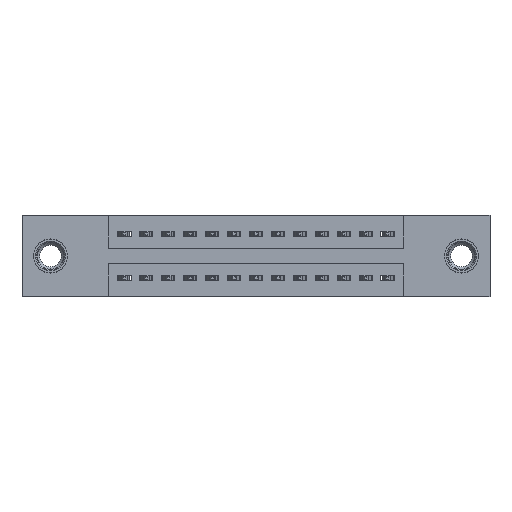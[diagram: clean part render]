
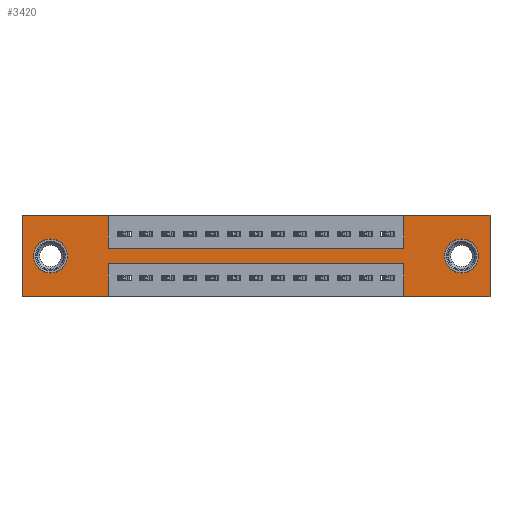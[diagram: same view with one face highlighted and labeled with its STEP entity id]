
A CAD part, front view. The second image highlights one B-rep face of the part: STEP entity #3420.
In plain terms, the highlighted planar face has unit normal (0, -1, 0).
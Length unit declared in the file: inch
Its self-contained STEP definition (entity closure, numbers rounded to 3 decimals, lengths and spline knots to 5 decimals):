
#12 = LINE ( 'NONE', #1189, #12251 ) ;
#26 = VECTOR ( 'NONE', #10800, 39.37008 ) ;
#217 = CARTESIAN_POINT ( 'NONE',  ( 0., 0., 0. ) ) ;
#230 = EDGE_CURVE ( 'NONE', #8303, #11624, #4557, .T. ) ;
#232 = ORIENTED_EDGE ( 'NONE', *, *, #5012, .F. ) ;
#518 = LINE ( 'NONE', #7254, #12726 ) ;
#530 = DIRECTION ( 'NONE',  ( -1., 0., 0. ) ) ;
#942 = CARTESIAN_POINT ( 'NONE',  ( 0.3925, 0., -0.22 ) ) ;
#1106 = VERTEX_POINT ( 'NONE', #10274 ) ;
#1141 = DIRECTION ( 'NONE',  ( 0., 0., -1. ) ) ;
#1189 = CARTESIAN_POINT ( 'NONE',  ( 1.7425, 0., 0. ) ) ;
#1346 = VERTEX_POINT ( 'NONE', #8448 ) ;
#1423 = VERTEX_POINT ( 'NONE', #8037 ) ;
#1599 = EDGE_CURVE ( 'NONE', #9933, #1677, #8602, .T. ) ;
#1677 = VERTEX_POINT ( 'NONE', #5876 ) ;
#1917 = CARTESIAN_POINT ( 'NONE',  ( 0.13, 0., -0.185 ) ) ;
#1989 = VERTEX_POINT ( 'NONE', #2842 ) ;
#2098 = ORIENTED_EDGE ( 'NONE', *, *, #14402, .F. ) ;
#2321 = EDGE_CURVE ( 'NONE', #1423, #8303, #8020, .T. ) ;
#2339 = EDGE_CURVE ( 'NONE', #1677, #9933, #11106, .T. ) ;
#2755 = DIRECTION ( 'NONE',  ( 0., 1., 0. ) ) ;
#2811 = ORIENTED_EDGE ( 'NONE', *, *, #11358, .F. ) ;
#2842 = CARTESIAN_POINT ( 'NONE',  ( 2.135, 0., -0.37 ) ) ;
#2963 = DIRECTION ( 'NONE',  ( 1., 0., 0. ) ) ;
#3110 = DIRECTION ( 'NONE',  ( 0., 0., 1. ) ) ;
#3420 = ADVANCED_FACE ( 'NONE', ( #13262, #4289, #10163 ), #3512, .T. ) ;
#3491 = AXIS2_PLACEMENT_3D ( 'NONE', #1917, #10160, #3110 ) ;
#3512 = PLANE ( 'NONE',  #15253 ) ;
#3604 = DIRECTION ( 'NONE',  ( 0., 0., 1. ) ) ;
#3617 = VERTEX_POINT ( 'NONE', #10950 ) ;
#3681 = CARTESIAN_POINT ( 'NONE',  ( 1.7425, 0., -0.22 ) ) ;
#3774 = EDGE_LOOP ( 'NONE', ( #9457, #4129 ) ) ;
#3805 = ORIENTED_EDGE ( 'NONE', *, *, #9025, .F. ) ;
#3922 = DIRECTION ( 'NONE',  ( 0., 0., -1. ) ) ;
#4040 = CARTESIAN_POINT ( 'NONE',  ( 1.7425, 0., -0.15 ) ) ;
#4041 = VECTOR ( 'NONE', #14000, 39.37008 ) ;
#4082 = CARTESIAN_POINT ( 'NONE',  ( 0., 0., 0. ) ) ;
#4129 = ORIENTED_EDGE ( 'NONE', *, *, #2339, .T. ) ;
#4289 = FACE_BOUND ( 'NONE', #5256, .T. ) ;
#4371 = AXIS2_PLACEMENT_3D ( 'NONE', #9816, #2755, #10982 ) ;
#4382 = VECTOR ( 'NONE', #5471, 39.37008 ) ;
#4389 = CARTESIAN_POINT ( 'NONE',  ( 0., 0., -0.37 ) ) ;
#4421 = DIRECTION ( 'NONE',  ( 0., 0., -1. ) ) ;
#4557 = LINE ( 'NONE', #6853, #10424 ) ;
#4796 = ORIENTED_EDGE ( 'NONE', *, *, #2321, .F. ) ;
#4852 = VERTEX_POINT ( 'NONE', #9800 ) ;
#5012 = EDGE_CURVE ( 'NONE', #4852, #1423, #7203, .T. ) ;
#5133 = ORIENTED_EDGE ( 'NONE', *, *, #12917, .F. ) ;
#5177 = VERTEX_POINT ( 'NONE', #10352 ) ;
#5256 = EDGE_LOOP ( 'NONE', ( #9571, #11284 ) ) ;
#5416 = EDGE_LOOP ( 'NONE', ( #12887, #5133, #2811, #7409, #2098, #5467, #7457, #3805, #9372, #7187, #4796, #232 ) ) ;
#5467 = ORIENTED_EDGE ( 'NONE', *, *, #10111, .F. ) ;
#5471 = DIRECTION ( 'NONE',  ( 0., 0., 1. ) ) ;
#5876 = CARTESIAN_POINT ( 'NONE',  ( 2.005, 0., -0.263 ) ) ;
#6128 = DIRECTION ( 'NONE',  ( 0., 0., -1. ) ) ;
#6266 = CARTESIAN_POINT ( 'NONE',  ( 0.13, 0., -0.185 ) ) ;
#6285 = DIRECTION ( 'NONE',  ( 0., 0., -1. ) ) ;
#6308 = DIRECTION ( 'NONE',  ( 0., 1., 0. ) ) ;
#6317 = CARTESIAN_POINT ( 'NONE',  ( 2.005, 0., -0.185 ) ) ;
#6533 = VECTOR ( 'NONE', #11842, 39.37008 ) ;
#6653 = CARTESIAN_POINT ( 'NONE',  ( 1.7425, 0., -0.37 ) ) ;
#6675 = VERTEX_POINT ( 'NONE', #942 ) ;
#6677 = VECTOR ( 'NONE', #2963, 39.37008 ) ;
#6799 = DIRECTION ( 'NONE',  ( 1., 0., 0. ) ) ;
#6853 = CARTESIAN_POINT ( 'NONE',  ( 0., 0., 0. ) ) ;
#6871 = CIRCLE ( 'NONE', #3491, 0.078 ) ;
#6905 = LINE ( 'NONE', #9526, #6533 ) ;
#7187 = ORIENTED_EDGE ( 'NONE', *, *, #230, .F. ) ;
#7189 = LINE ( 'NONE', #4389, #4041 ) ;
#7203 = LINE ( 'NONE', #14732, #13020 ) ;
#7254 = CARTESIAN_POINT ( 'NONE',  ( 0.3925, 0., 0. ) ) ;
#7409 = ORIENTED_EDGE ( 'NONE', *, *, #10504, .F. ) ;
#7411 = VERTEX_POINT ( 'NONE', #3681 ) ;
#7448 = DIRECTION ( 'NONE',  ( 0., 0., 1. ) ) ;
#7457 = ORIENTED_EDGE ( 'NONE', *, *, #10588, .F. ) ;
#7472 = EDGE_CURVE ( 'NONE', #11624, #9283, #518, .T. ) ;
#7780 = VECTOR ( 'NONE', #3922, 39.37008 ) ;
#7931 = CARTESIAN_POINT ( 'NONE',  ( 0.3925, 0., -0.37 ) ) ;
#8020 = LINE ( 'NONE', #217, #12175 ) ;
#8037 = CARTESIAN_POINT ( 'NONE',  ( 0., 0., -0.37 ) ) ;
#8189 = EDGE_CURVE ( 'NONE', #5177, #1346, #11790, .T. ) ;
#8271 = DIRECTION ( 'NONE',  ( 0., -1., 0. ) ) ;
#8303 = VERTEX_POINT ( 'NONE', #4082 ) ;
#8448 = CARTESIAN_POINT ( 'NONE',  ( 0.13, 0., -0.107 ) ) ;
#8602 = CIRCLE ( 'NONE', #12274, 0.078 ) ;
#9025 = EDGE_CURVE ( 'NONE', #9283, #12463, #10150, .T. ) ;
#9283 = VERTEX_POINT ( 'NONE', #10471 ) ;
#9372 = ORIENTED_EDGE ( 'NONE', *, *, #7472, .F. ) ;
#9457 = ORIENTED_EDGE ( 'NONE', *, *, #1599, .T. ) ;
#9526 = CARTESIAN_POINT ( 'NONE',  ( 0.3925, 0., -0.22 ) ) ;
#9571 = ORIENTED_EDGE ( 'NONE', *, *, #13810, .T. ) ;
#9641 = CARTESIAN_POINT ( 'NONE',  ( 0., 0., 0. ) ) ;
#9800 = CARTESIAN_POINT ( 'NONE',  ( 0.3925, 0., -0.37 ) ) ;
#9816 = CARTESIAN_POINT ( 'NONE',  ( 2.005, 0., -0.185 ) ) ;
#9933 = VERTEX_POINT ( 'NONE', #10455 ) ;
#10106 = VECTOR ( 'NONE', #4421, 39.37008 ) ;
#10111 = EDGE_CURVE ( 'NONE', #1106, #11264, #12636, .T. ) ;
#10115 = AXIS2_PLACEMENT_3D ( 'NONE', #6266, #14411, #7448 ) ;
#10150 = LINE ( 'NONE', #11189, #6677 ) ;
#10160 = DIRECTION ( 'NONE',  ( 0., 1., 0. ) ) ;
#10163 = FACE_OUTER_BOUND ( 'NONE', #5416, .T. ) ;
#10274 = CARTESIAN_POINT ( 'NONE',  ( 1.7425, 0., 0. ) ) ;
#10352 = CARTESIAN_POINT ( 'NONE',  ( 0.13, 0., -0.263 ) ) ;
#10424 = VECTOR ( 'NONE', #6799, 39.37008 ) ;
#10455 = CARTESIAN_POINT ( 'NONE',  ( 2.005, 0., -0.107 ) ) ;
#10471 = CARTESIAN_POINT ( 'NONE',  ( 0.3925, 0., -0.15 ) ) ;
#10504 = EDGE_CURVE ( 'NONE', #1989, #3617, #7189, .T. ) ;
#10588 = EDGE_CURVE ( 'NONE', #12463, #1106, #12, .T. ) ;
#10678 = CARTESIAN_POINT ( 'NONE',  ( 2.135, 0., 0. ) ) ;
#10682 = CARTESIAN_POINT ( 'NONE',  ( 0.3925, 0., 0. ) ) ;
#10800 = DIRECTION ( 'NONE',  ( 1., 0., 0. ) ) ;
#10864 = LINE ( 'NONE', #10942, #7780 ) ;
#10942 = CARTESIAN_POINT ( 'NONE',  ( 2.135, 0., 0. ) ) ;
#10950 = CARTESIAN_POINT ( 'NONE',  ( 1.7425, 0., -0.37 ) ) ;
#10982 = DIRECTION ( 'NONE',  ( 0., 0., -1. ) ) ;
#11106 = CIRCLE ( 'NONE', #4371, 0.078 ) ;
#11189 = CARTESIAN_POINT ( 'NONE',  ( 0.3925, 0., -0.15 ) ) ;
#11264 = VERTEX_POINT ( 'NONE', #10678 ) ;
#11284 = ORIENTED_EDGE ( 'NONE', *, *, #8189, .T. ) ;
#11358 = EDGE_CURVE ( 'NONE', #3617, #7411, #13708, .T. ) ;
#11624 = VERTEX_POINT ( 'NONE', #10682 ) ;
#11790 = CIRCLE ( 'NONE', #10115, 0.078 ) ;
#11842 = DIRECTION ( 'NONE',  ( -1., 0., 0. ) ) ;
#12034 = DIRECTION ( 'NONE',  ( 0., 0., 1. ) ) ;
#12175 = VECTOR ( 'NONE', #12034, 39.37008 ) ;
#12251 = VECTOR ( 'NONE', #3604, 39.37008 ) ;
#12274 = AXIS2_PLACEMENT_3D ( 'NONE', #6317, #6308, #6285 ) ;
#12463 = VERTEX_POINT ( 'NONE', #4040 ) ;
#12636 = LINE ( 'NONE', #9641, #26 ) ;
#12726 = VECTOR ( 'NONE', #6128, 39.37008 ) ;
#12887 = ORIENTED_EDGE ( 'NONE', *, *, #15267, .F. ) ;
#12917 = EDGE_CURVE ( 'NONE', #7411, #6675, #6905, .T. ) ;
#13020 = VECTOR ( 'NONE', #530, 39.37008 ) ;
#13209 = LINE ( 'NONE', #7931, #10106 ) ;
#13262 = FACE_BOUND ( 'NONE', #3774, .T. ) ;
#13708 = LINE ( 'NONE', #6653, #4382 ) ;
#13810 = EDGE_CURVE ( 'NONE', #1346, #5177, #6871, .T. ) ;
#14000 = DIRECTION ( 'NONE',  ( -1., 0., 0. ) ) ;
#14402 = EDGE_CURVE ( 'NONE', #11264, #1989, #10864, .T. ) ;
#14411 = DIRECTION ( 'NONE',  ( 0., 1., 0. ) ) ;
#14732 = CARTESIAN_POINT ( 'NONE',  ( 0., 0., -0.37 ) ) ;
#15238 = CARTESIAN_POINT ( 'NONE',  ( 0., 0., -0.37 ) ) ;
#15253 = AXIS2_PLACEMENT_3D ( 'NONE', #15238, #8271, #1141 ) ;
#15267 = EDGE_CURVE ( 'NONE', #6675, #4852, #13209, .T. ) ;
